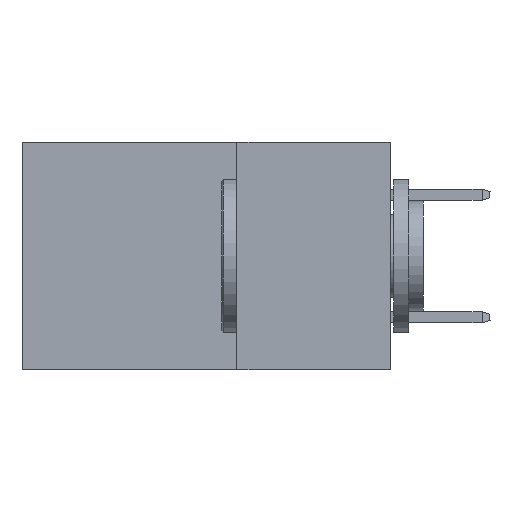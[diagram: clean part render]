
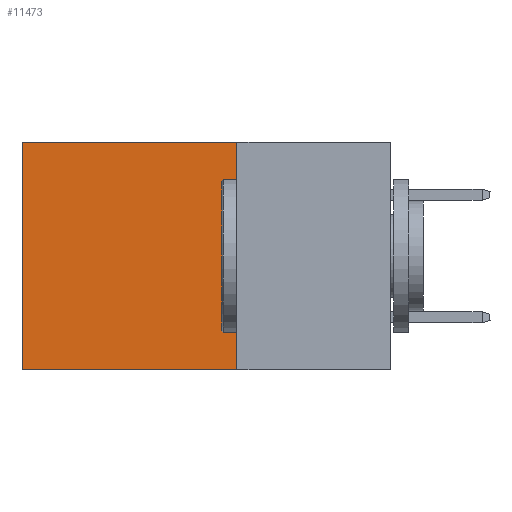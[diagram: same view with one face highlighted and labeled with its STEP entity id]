
A CAD part, left-side view. The second image highlights one B-rep face of the part: STEP entity #11473.
In plain terms, the highlighted planar face has unit normal (-1, 0, 0).
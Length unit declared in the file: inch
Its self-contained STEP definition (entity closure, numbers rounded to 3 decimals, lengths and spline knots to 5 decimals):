
#279 = DIRECTION ( 'NONE',  ( 0., 1., 0. ) ) ;
#695 = ORIENTED_EDGE ( 'NONE', *, *, #7120, .T. ) ;
#1680 = AXIS2_PLACEMENT_3D ( 'NONE', #7566, #5979, #1724 ) ;
#1724 = DIRECTION ( 'NONE',  ( 0., 0., -1. ) ) ;
#2472 = EDGE_CURVE ( 'NONE', #6177, #3066, #13640, .T. ) ;
#2715 = FACE_OUTER_BOUND ( 'NONE', #14508, .T. ) ;
#3066 = VERTEX_POINT ( 'NONE', #14576 ) ;
#3741 = LINE ( 'NONE', #9570, #7411 ) ;
#4307 = CARTESIAN_POINT ( 'NONE',  ( 0.2875, 0.25, 0. ) ) ;
#5787 = CARTESIAN_POINT ( 'NONE',  ( 0.2875, 0.25, -0.37 ) ) ;
#5979 = DIRECTION ( 'NONE',  ( 1., 0., 0. ) ) ;
#6177 = VERTEX_POINT ( 'NONE', #5787 ) ;
#7120 = EDGE_CURVE ( 'NONE', #17831, #18504, #17717, .T. ) ;
#7411 = VECTOR ( 'NONE', #13978, 39.37008 ) ;
#7425 = DIRECTION ( 'NONE',  ( 0., 0., -1. ) ) ;
#7566 = CARTESIAN_POINT ( 'NONE',  ( 0.2875, 0.25, 0. ) ) ;
#7651 = CARTESIAN_POINT ( 'NONE',  ( 0.2875, 0.25, -0.37 ) ) ;
#9570 = CARTESIAN_POINT ( 'NONE',  ( 0.2875, 0.25, 0. ) ) ;
#9779 = VECTOR ( 'NONE', #279, 39.37008 ) ;
#9933 = CARTESIAN_POINT ( 'NONE',  ( 0.2875, 0.6, 0. ) ) ;
#10713 = CARTESIAN_POINT ( 'NONE',  ( 0.2875, 0.6, 0. ) ) ;
#11473 = ADVANCED_FACE ( 'NONE', ( #2715 ), #16267, .F. ) ;
#12713 = ORIENTED_EDGE ( 'NONE', *, *, #2472, .F. ) ;
#12933 = CARTESIAN_POINT ( 'NONE',  ( 0.2875, 0.25, 0. ) ) ;
#13640 = LINE ( 'NONE', #7651, #9779 ) ;
#13713 = LINE ( 'NONE', #9933, #15066 ) ;
#13978 = DIRECTION ( 'NONE',  ( 0., 0., -1. ) ) ;
#14418 = DIRECTION ( 'NONE',  ( 0., 1., 0. ) ) ;
#14508 = EDGE_LOOP ( 'NONE', ( #15258, #12713, #15598, #695 ) ) ;
#14576 = CARTESIAN_POINT ( 'NONE',  ( 0.2875, 0.6, -0.37 ) ) ;
#15066 = VECTOR ( 'NONE', #7425, 39.37008 ) ;
#15258 = ORIENTED_EDGE ( 'NONE', *, *, #17744, .T. ) ;
#15598 = ORIENTED_EDGE ( 'NONE', *, *, #17509, .F. ) ;
#16267 = PLANE ( 'NONE',  #1680 ) ;
#16810 = VECTOR ( 'NONE', #14418, 39.37008 ) ;
#17509 = EDGE_CURVE ( 'NONE', #17831, #6177, #3741, .T. ) ;
#17717 = LINE ( 'NONE', #4307, #16810 ) ;
#17744 = EDGE_CURVE ( 'NONE', #18504, #3066, #13713, .T. ) ;
#17831 = VERTEX_POINT ( 'NONE', #12933 ) ;
#18504 = VERTEX_POINT ( 'NONE', #10713 ) ;
